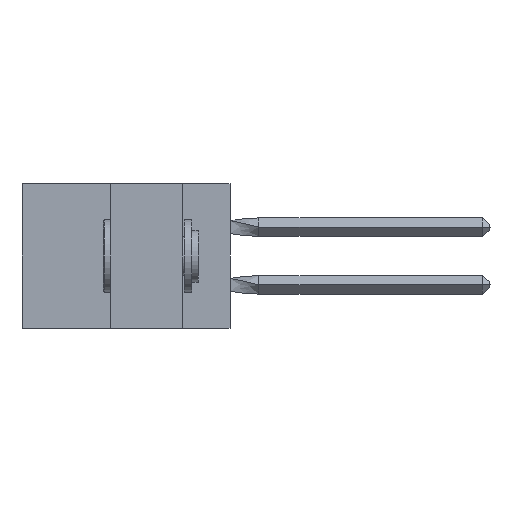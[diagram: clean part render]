
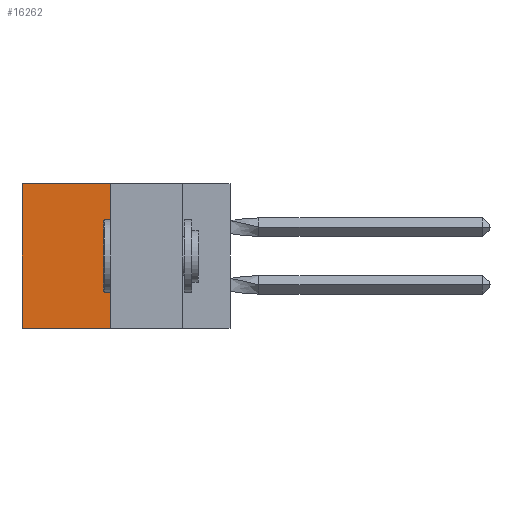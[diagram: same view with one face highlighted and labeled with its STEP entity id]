
A CAD part, left-side view. The second image highlights one B-rep face of the part: STEP entity #16262.
In plain terms, the highlighted planar face has unit normal (-1, 0, 0).
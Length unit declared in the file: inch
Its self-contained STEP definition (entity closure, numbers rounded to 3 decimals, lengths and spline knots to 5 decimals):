
#221 = VECTOR ( 'NONE', #15003, 39.37008 ) ;
#1964 = VERTEX_POINT ( 'NONE', #17331 ) ;
#3159 = CARTESIAN_POINT ( 'NONE',  ( 0.305, 0.72, -0.5 ) ) ;
#3235 = ORIENTED_EDGE ( 'NONE', *, *, #16605, .F. ) ;
#6125 = DIRECTION ( 'NONE',  ( 0., 0., -1. ) ) ;
#8846 = VECTOR ( 'NONE', #27856, 39.37008 ) ;
#11018 = LINE ( 'NONE', #21794, #8846 ) ;
#11369 = VERTEX_POINT ( 'NONE', #3159 ) ;
#12259 = EDGE_LOOP ( 'NONE', ( #15813, #18542, #3235, #21450 ) ) ;
#15003 = DIRECTION ( 'NONE',  ( 0., 1., 0. ) ) ;
#15031 = CARTESIAN_POINT ( 'NONE',  ( 0.305, 0.413, -0.5 ) ) ;
#15516 = CARTESIAN_POINT ( 'NONE',  ( 0.305, 0.72, 0. ) ) ;
#15813 = ORIENTED_EDGE ( 'NONE', *, *, #27279, .T. ) ;
#16262 = ADVANCED_FACE ( 'NONE', ( #29426 ), #24057, .F. ) ;
#16605 = EDGE_CURVE ( 'NONE', #1964, #31562, #25394, .T. ) ;
#17331 = CARTESIAN_POINT ( 'NONE',  ( 0.305, 0.413, 0. ) ) ;
#17891 = LINE ( 'NONE', #28902, #221 ) ;
#18542 = ORIENTED_EDGE ( 'NONE', *, *, #19634, .F. ) ;
#18545 = DIRECTION ( 'NONE',  ( 0., 0., -1. ) ) ;
#19634 = EDGE_CURVE ( 'NONE', #31562, #11369, #11018, .T. ) ;
#20408 = VECTOR ( 'NONE', #6125, 39.37008 ) ;
#21337 = VECTOR ( 'NONE', #31745, 39.37008 ) ;
#21450 = ORIENTED_EDGE ( 'NONE', *, *, #22575, .T. ) ;
#21794 = CARTESIAN_POINT ( 'NONE',  ( 0.305, 0.413, -0.5 ) ) ;
#22575 = EDGE_CURVE ( 'NONE', #1964, #31937, #17891, .T. ) ;
#24057 = PLANE ( 'NONE',  #29829 ) ;
#25394 = LINE ( 'NONE', #15031, #21337 ) ;
#25947 = CARTESIAN_POINT ( 'NONE',  ( 0.305, 0.413, -0.5 ) ) ;
#26895 = DIRECTION ( 'NONE',  ( 1., 0., 0. ) ) ;
#27279 = EDGE_CURVE ( 'NONE', #31937, #11369, #29657, .T. ) ;
#27856 = DIRECTION ( 'NONE',  ( 0., 1., 0. ) ) ;
#28902 = CARTESIAN_POINT ( 'NONE',  ( 0.305, 0.413, 0. ) ) ;
#29426 = FACE_OUTER_BOUND ( 'NONE', #12259, .T. ) ;
#29657 = LINE ( 'NONE', #34482, #20408 ) ;
#29829 = AXIS2_PLACEMENT_3D ( 'NONE', #32700, #26895, #18545 ) ;
#31562 = VERTEX_POINT ( 'NONE', #25947 ) ;
#31745 = DIRECTION ( 'NONE',  ( 0., 0., -1. ) ) ;
#31937 = VERTEX_POINT ( 'NONE', #15516 ) ;
#32700 = CARTESIAN_POINT ( 'NONE',  ( 0.305, 0.413, -0.5 ) ) ;
#34482 = CARTESIAN_POINT ( 'NONE',  ( 0.305, 0.72, -0.5 ) ) ;
